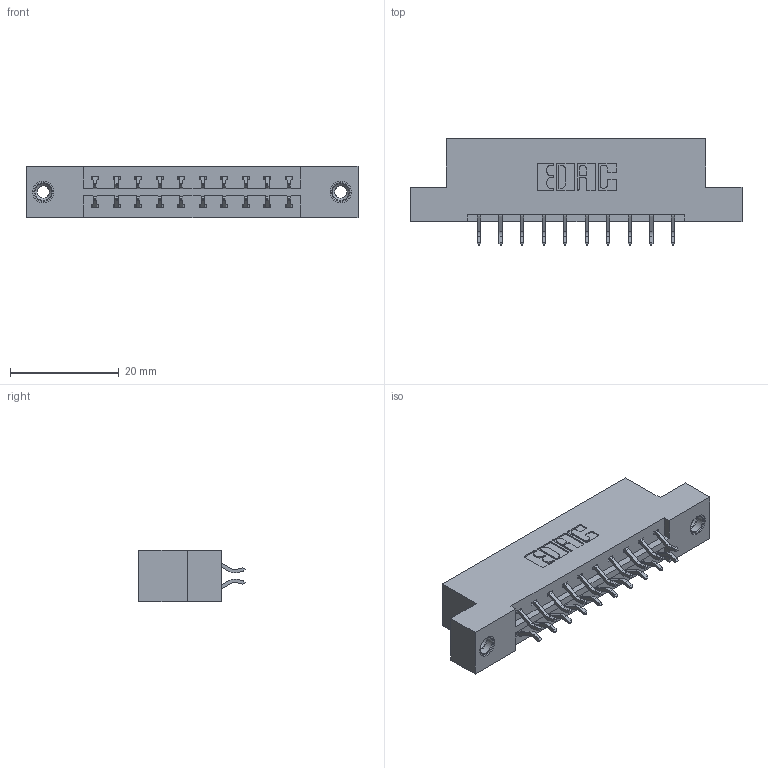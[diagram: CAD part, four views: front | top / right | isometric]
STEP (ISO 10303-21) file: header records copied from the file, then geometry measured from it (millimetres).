
FILE_DESCRIPTION (( 'STEP AP203' ), '1' );
FILE_NAME ('833-020-556-208.STEP', '2020-06-01T13:47:47', ( '' ), ( '' ), 'SwSTEP 2.0', 'SolidWorks 2020', '' );
FILE_SCHEMA (( 'CONFIG_CONTROL_DESIGN' ));
Length unit declared in the file: inch
Products named in the file (4): 345-292-001_556 Tail; 833-020-556-208; 345-250-001_345-250-003-102; 833 Part_Flush - .156 Dia - TI
Assembly tree (23 placements, depth 2):
  833-020-556-208
    833 Part_Flush - .156 Dia - TI
    345-292-001_556 Tail  x20
    345-250-001_345-250-003-102  x2
Bounding box: 61.16 x 19.57 x 9.4 mm (x, y, z)
Volume: 5937.8 mm3; surface area: 6678.2 mm2
Topology: 23 solids, 23 shells, 1334 faces, 3907 edges, 2570 vertices
Faces by surface type: plane 902, cylinder 416, cone 12, torus 4
Entity records: 11978 total; most frequent: CARTESIAN_POINT 2021, ORIENTED_EDGE 1938, DIRECTION 1803, EDGE_CURVE 969, VECTOR 813, LINE 813, VERTEX_POINT 640, AXIS2_PLACEMENT_3D 495
